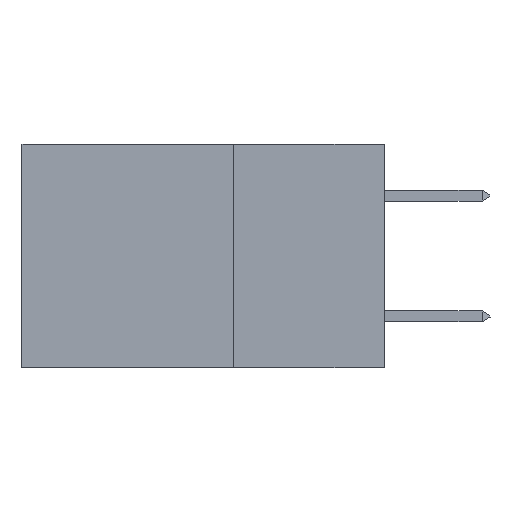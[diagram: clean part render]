
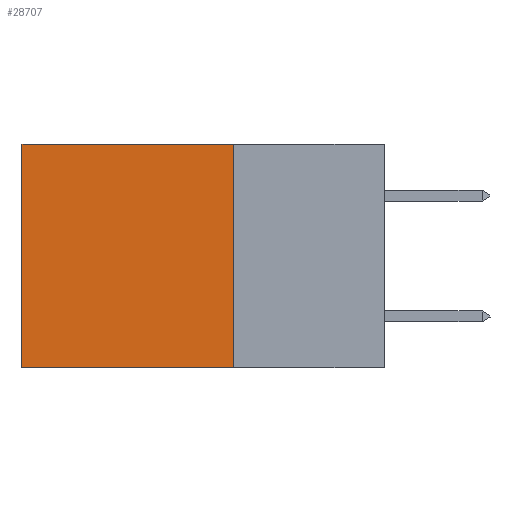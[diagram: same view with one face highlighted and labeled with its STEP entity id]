
A CAD part, left-side view. The second image highlights one B-rep face of the part: STEP entity #28707.
In plain terms, the highlighted planar face has unit normal (-1, 0, 0).
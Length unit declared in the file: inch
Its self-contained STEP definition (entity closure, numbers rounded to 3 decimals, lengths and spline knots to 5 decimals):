
#2082 = VERTEX_POINT ( 'NONE', #4616 ) ;
#2118 = DIRECTION ( 'NONE',  ( 0., 1., 0. ) ) ;
#2756 = CARTESIAN_POINT ( 'NONE',  ( 0.2875, 0.6, 0. ) ) ;
#3561 = VECTOR ( 'NONE', #16450, 39.37008 ) ;
#4334 = AXIS2_PLACEMENT_3D ( 'NONE', #7385, #25725, #11970 ) ;
#4616 = CARTESIAN_POINT ( 'NONE',  ( 0.2875, 0.6, -0.37 ) ) ;
#6874 = VERTEX_POINT ( 'NONE', #18870 ) ;
#7385 = CARTESIAN_POINT ( 'NONE',  ( 0.2875, 0.25, 0. ) ) ;
#7796 = DIRECTION ( 'NONE',  ( 0., 0., -1. ) ) ;
#8925 = ORIENTED_EDGE ( 'NONE', *, *, #11302, .T. ) ;
#9337 = FACE_OUTER_BOUND ( 'NONE', #16710, .T. ) ;
#9735 = CARTESIAN_POINT ( 'NONE',  ( 0.2875, 0.25, 0. ) ) ;
#10676 = DIRECTION ( 'NONE',  ( 0., 1., 0. ) ) ;
#10762 = EDGE_CURVE ( 'NONE', #6874, #2082, #23921, .T. ) ;
#11302 = EDGE_CURVE ( 'NONE', #22819, #27635, #16360, .T. ) ;
#11970 = DIRECTION ( 'NONE',  ( 0., 0., -1. ) ) ;
#13008 = CARTESIAN_POINT ( 'NONE',  ( 0.2875, 0.25, 0. ) ) ;
#14618 = ORIENTED_EDGE ( 'NONE', *, *, #25591, .F. ) ;
#15639 = VECTOR ( 'NONE', #10676, 39.37008 ) ;
#16360 = LINE ( 'NONE', #13008, #15639 ) ;
#16450 = DIRECTION ( 'NONE',  ( 0., 0., -1. ) ) ;
#16710 = EDGE_LOOP ( 'NONE', ( #25234, #20567, #14618, #8925 ) ) ;
#17061 = LINE ( 'NONE', #28323, #28559 ) ;
#18870 = CARTESIAN_POINT ( 'NONE',  ( 0.2875, 0.25, -0.37 ) ) ;
#20567 = ORIENTED_EDGE ( 'NONE', *, *, #10762, .F. ) ;
#21064 = PLANE ( 'NONE',  #4334 ) ;
#22542 = CARTESIAN_POINT ( 'NONE',  ( 0.2875, 0.6, 0. ) ) ;
#22819 = VERTEX_POINT ( 'NONE', #9735 ) ;
#23921 = LINE ( 'NONE', #27243, #24663 ) ;
#24663 = VECTOR ( 'NONE', #2118, 39.37008 ) ;
#25234 = ORIENTED_EDGE ( 'NONE', *, *, #29317, .T. ) ;
#25591 = EDGE_CURVE ( 'NONE', #22819, #6874, #17061, .T. ) ;
#25725 = DIRECTION ( 'NONE',  ( 1., 0., 0. ) ) ;
#27243 = CARTESIAN_POINT ( 'NONE',  ( 0.2875, 0.25, -0.37 ) ) ;
#27635 = VERTEX_POINT ( 'NONE', #22542 ) ;
#27937 = LINE ( 'NONE', #2756, #3561 ) ;
#28323 = CARTESIAN_POINT ( 'NONE',  ( 0.2875, 0.25, 0. ) ) ;
#28559 = VECTOR ( 'NONE', #7796, 39.37008 ) ;
#28707 = ADVANCED_FACE ( 'NONE', ( #9337 ), #21064, .F. ) ;
#29317 = EDGE_CURVE ( 'NONE', #27635, #2082, #27937, .T. ) ;
